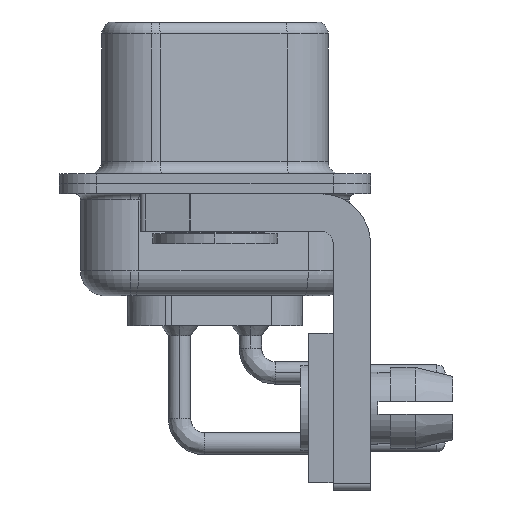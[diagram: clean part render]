
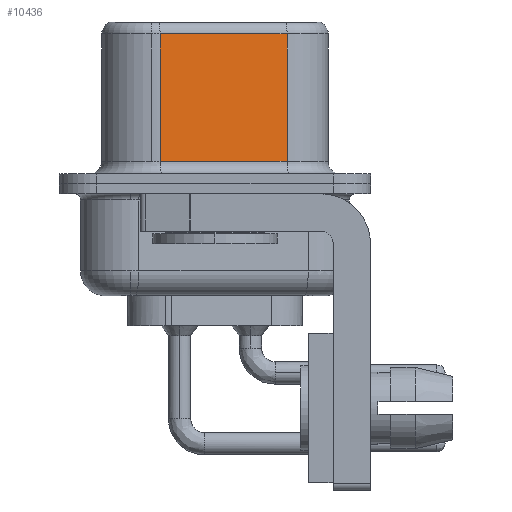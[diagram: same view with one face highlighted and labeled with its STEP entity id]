
A CAD part, left-side view. The second image highlights one B-rep face of the part: STEP entity #10436.
In plain terms, the highlighted planar face has unit normal (-0.985, -0.174, 0).
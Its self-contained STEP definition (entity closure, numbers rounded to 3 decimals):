
#120 = LINE ( 'NONE', #22228, #20865 ) ;
#156 = DIRECTION ( 'NONE',  ( 0.174, -0.985, 0. ) ) ;
#2210 = CARTESIAN_POINT ( 'NONE',  ( 4.555, -2.897, 0.9 ) ) ;
#3567 = CARTESIAN_POINT ( 'NONE',  ( 3.655, 2.203, 6.02 ) ) ;
#4346 = FACE_OUTER_BOUND ( 'NONE', #21678, .T. ) ;
#4642 = EDGE_CURVE ( 'NONE', #13727, #15747, #24993, .T. ) ;
#4690 = ORIENTED_EDGE ( 'NONE', *, *, #14167, .T. ) ;
#5861 = EDGE_CURVE ( 'NONE', #22852, #6544, #120, .T. ) ;
#6291 = DIRECTION ( 'NONE',  ( 0., 0., -1. ) ) ;
#6544 = VERTEX_POINT ( 'NONE', #20849 ) ;
#8203 = DIRECTION ( 'NONE',  ( 0., 0., -1. ) ) ;
#9212 = LINE ( 'NONE', #2210, #24567 ) ;
#9750 = CARTESIAN_POINT ( 'NONE',  ( 4.555, -2.897, 6.52 ) ) ;
#10245 = CARTESIAN_POINT ( 'NONE',  ( 3.655, 2.203, 6.52 ) ) ;
#10436 = ADVANCED_FACE ( 'NONE', ( #4346 ), #11702, .F. ) ;
#11702 = PLANE ( 'NONE',  #25339 ) ;
#11786 = DIRECTION ( 'NONE',  ( -0.174, 0.985, 0. ) ) ;
#12442 = CARTESIAN_POINT ( 'NONE',  ( 4.555, -2.897, 6.02 ) ) ;
#13459 = ORIENTED_EDGE ( 'NONE', *, *, #4642, .T. ) ;
#13460 = CARTESIAN_POINT ( 'NONE',  ( 4.555, -2.897, 6.02 ) ) ;
#13727 = VERTEX_POINT ( 'NONE', #3567 ) ;
#14167 = EDGE_CURVE ( 'NONE', #15747, #6544, #9212, .T. ) ;
#15621 = VECTOR ( 'NONE', #8203, 1000. ) ;
#15747 = VERTEX_POINT ( 'NONE', #21371 ) ;
#15871 = VECTOR ( 'NONE', #24241, 1000. ) ;
#16496 = LINE ( 'NONE', #12442, #15871 ) ;
#20849 = CARTESIAN_POINT ( 'NONE',  ( 4.555, -2.897, 0.9 ) ) ;
#20865 = VECTOR ( 'NONE', #6291, 1000. ) ;
#21371 = CARTESIAN_POINT ( 'NONE',  ( 3.655, 2.203, 0.9 ) ) ;
#21486 = EDGE_CURVE ( 'NONE', #22852, #13727, #16496, .T. ) ;
#21678 = EDGE_LOOP ( 'NONE', ( #24249, #24323, #13459, #4690 ) ) ;
#22228 = CARTESIAN_POINT ( 'NONE',  ( 4.555, -2.897, 6.52 ) ) ;
#22852 = VERTEX_POINT ( 'NONE', #13460 ) ;
#23751 = DIRECTION ( 'NONE',  ( 0.985, 0.174, 0. ) ) ;
#24241 = DIRECTION ( 'NONE',  ( -0.174, 0.985, 0. ) ) ;
#24249 = ORIENTED_EDGE ( 'NONE', *, *, #5861, .F. ) ;
#24323 = ORIENTED_EDGE ( 'NONE', *, *, #21486, .T. ) ;
#24567 = VECTOR ( 'NONE', #156, 1000. ) ;
#24993 = LINE ( 'NONE', #10245, #15621 ) ;
#25339 = AXIS2_PLACEMENT_3D ( 'NONE', #9750, #23751, #11786 ) ;
